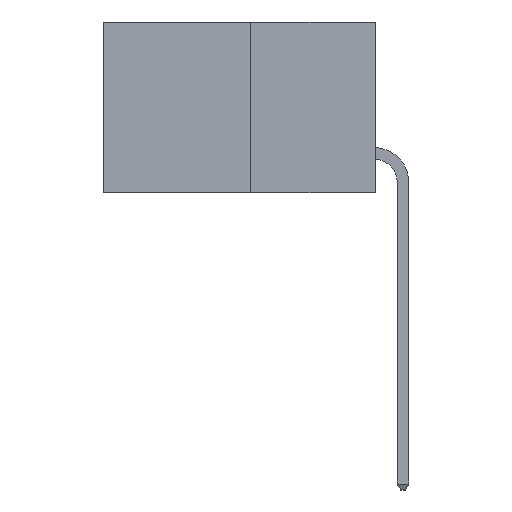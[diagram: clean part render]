
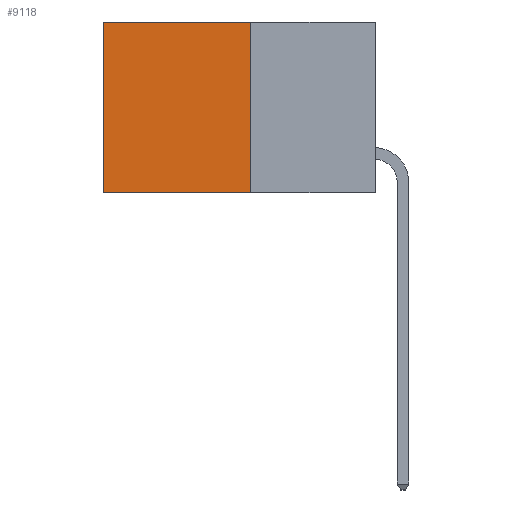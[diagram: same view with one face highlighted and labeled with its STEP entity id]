
A CAD part, left-side view. The second image highlights one B-rep face of the part: STEP entity #9118.
In plain terms, the highlighted planar face has unit normal (-1, 0, 0).
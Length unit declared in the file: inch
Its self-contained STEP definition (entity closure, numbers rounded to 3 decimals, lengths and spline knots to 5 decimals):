
#386 = VECTOR ( 'NONE', #9076, 39.37008 ) ;
#448 = VERTEX_POINT ( 'NONE', #9880 ) ;
#682 = AXIS2_PLACEMENT_3D ( 'NONE', #2253, #8429, #3145 ) ;
#888 = EDGE_LOOP ( 'NONE', ( #3991, #2894, #1537, #8039 ) ) ;
#1127 = CARTESIAN_POINT ( 'NONE',  ( 0.277, 0.59, -0.37 ) ) ;
#1140 = VECTOR ( 'NONE', #8868, 39.37008 ) ;
#1537 = ORIENTED_EDGE ( 'NONE', *, *, #5546, .F. ) ;
#2253 = CARTESIAN_POINT ( 'NONE',  ( 0.277, 0.27, -0.37 ) ) ;
#2362 = CARTESIAN_POINT ( 'NONE',  ( 0.277, 0.59, -0.37 ) ) ;
#2605 = LINE ( 'NONE', #4513, #2889 ) ;
#2889 = VECTOR ( 'NONE', #6245, 39.37008 ) ;
#2894 = ORIENTED_EDGE ( 'NONE', *, *, #3582, .F. ) ;
#3145 = DIRECTION ( 'NONE',  ( 0., 0., -1. ) ) ;
#3582 = EDGE_CURVE ( 'NONE', #448, #7440, #2605, .T. ) ;
#3827 = DIRECTION ( 'NONE',  ( 0., 0., -1. ) ) ;
#3991 = ORIENTED_EDGE ( 'NONE', *, *, #6505, .T. ) ;
#4031 = LINE ( 'NONE', #7962, #1140 ) ;
#4139 = VECTOR ( 'NONE', #3827, 39.37008 ) ;
#4411 = LINE ( 'NONE', #9115, #4139 ) ;
#4513 = CARTESIAN_POINT ( 'NONE',  ( 0.277, 0.27, -0.37 ) ) ;
#5546 = EDGE_CURVE ( 'NONE', #5912, #448, #4411, .T. ) ;
#5912 = VERTEX_POINT ( 'NONE', #8697 ) ;
#6245 = DIRECTION ( 'NONE',  ( 0., 1., 0. ) ) ;
#6505 = EDGE_CURVE ( 'NONE', #10331, #7440, #10053, .T. ) ;
#6634 = PLANE ( 'NONE',  #682 ) ;
#7440 = VERTEX_POINT ( 'NONE', #2362 ) ;
#7962 = CARTESIAN_POINT ( 'NONE',  ( 0.277, 0.27, 0. ) ) ;
#8039 = ORIENTED_EDGE ( 'NONE', *, *, #10583, .T. ) ;
#8429 = DIRECTION ( 'NONE',  ( 1., 0., 0. ) ) ;
#8697 = CARTESIAN_POINT ( 'NONE',  ( 0.277, 0.27, 0. ) ) ;
#8868 = DIRECTION ( 'NONE',  ( 0., 1., 0. ) ) ;
#9076 = DIRECTION ( 'NONE',  ( 0., 0., -1. ) ) ;
#9115 = CARTESIAN_POINT ( 'NONE',  ( 0.277, 0.27, -0.37 ) ) ;
#9118 = ADVANCED_FACE ( 'NONE', ( #9599 ), #6634, .F. ) ;
#9365 = CARTESIAN_POINT ( 'NONE',  ( 0.277, 0.59, 0. ) ) ;
#9599 = FACE_OUTER_BOUND ( 'NONE', #888, .T. ) ;
#9880 = CARTESIAN_POINT ( 'NONE',  ( 0.277, 0.27, -0.37 ) ) ;
#10053 = LINE ( 'NONE', #1127, #386 ) ;
#10331 = VERTEX_POINT ( 'NONE', #9365 ) ;
#10583 = EDGE_CURVE ( 'NONE', #5912, #10331, #4031, .T. ) ;
